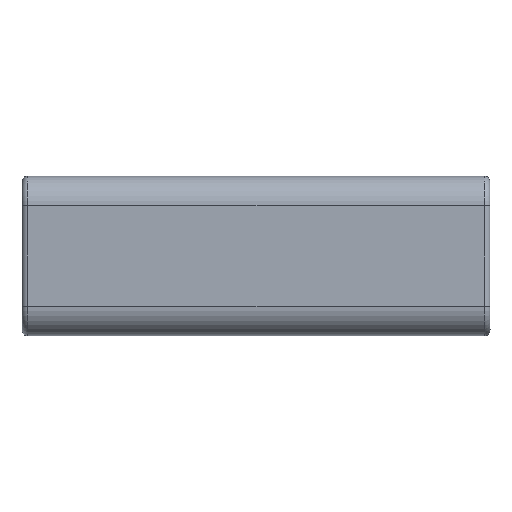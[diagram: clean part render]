
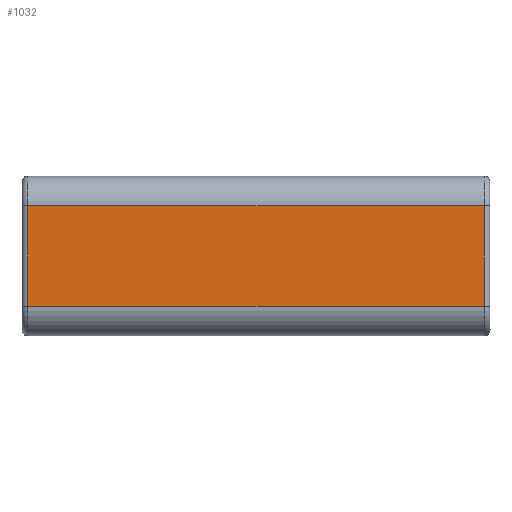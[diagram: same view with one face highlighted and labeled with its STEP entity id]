
A CAD part, front view. The second image highlights one B-rep face of the part: STEP entity #1032.
In plain terms, the highlighted planar face has unit normal (0, -1, 0).
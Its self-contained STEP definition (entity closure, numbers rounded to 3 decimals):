
#32=PLANE('',#1124);
#72=LINE('',#1627,#152);
#100=LINE('',#1695,#180);
#101=LINE('',#1699,#181);
#102=LINE('',#1700,#182);
#152=VECTOR('',#1269,10.);
#180=VECTOR('',#1335,10.);
#181=VECTOR('',#1340,10.);
#182=VECTOR('',#1341,10.);
#272=FACE_OUTER_BOUND('',#337,.T.);
#337=EDGE_LOOP('',(#796,#797,#798,#799));
#465=VERTEX_POINT('',#1619);
#467=VERTEX_POINT('',#1625);
#488=VERTEX_POINT('',#1694);
#489=VERTEX_POINT('',#1698);
#565=EDGE_CURVE('',#467,#465,#72,.T.);
#600=EDGE_CURVE('',#465,#488,#100,.T.);
#602=EDGE_CURVE('',#489,#467,#101,.T.);
#603=EDGE_CURVE('',#488,#489,#102,.T.);
#796=ORIENTED_EDGE('',*,*,#602,.F.);
#797=ORIENTED_EDGE('',*,*,#603,.F.);
#798=ORIENTED_EDGE('',*,*,#600,.F.);
#799=ORIENTED_EDGE('',*,*,#565,.F.);
#1032=ADVANCED_FACE('',(#272),#32,.T.);
#1124=AXIS2_PLACEMENT_3D('',#1697,#1338,#1339);
#1269=DIRECTION('',(0.,0.,1.));
#1335=DIRECTION('',(1.,0.,0.));
#1338=DIRECTION('center_axis',(0.,-1.,
0.));
#1339=DIRECTION('ref_axis',(0.,0.,1.));
#1340=DIRECTION('',(-1.,0.,0.));
#1341=DIRECTION('',(0.,0.,-1.));
#1619=CARTESIAN_POINT('',(41.05,129.447,-11.24));
#1625=CARTESIAN_POINT('',(41.05,129.447,-28.173));
#1627=CARTESIAN_POINT('',(41.05,129.447,-26.439));
#1694=CARTESIAN_POINT('',(118.018,129.447,-11.24));
#1695=CARTESIAN_POINT('',(149.018,129.447,-11.24));
#1697=CARTESIAN_POINT('Origin',(148.018,129.447,-33.173));
#1698=CARTESIAN_POINT('',(118.018,129.447,-28.173));
#1699=CARTESIAN_POINT('',(148.018,129.447,-28.173));
#1700=CARTESIAN_POINT('',(118.018,129.447,-26.439));
